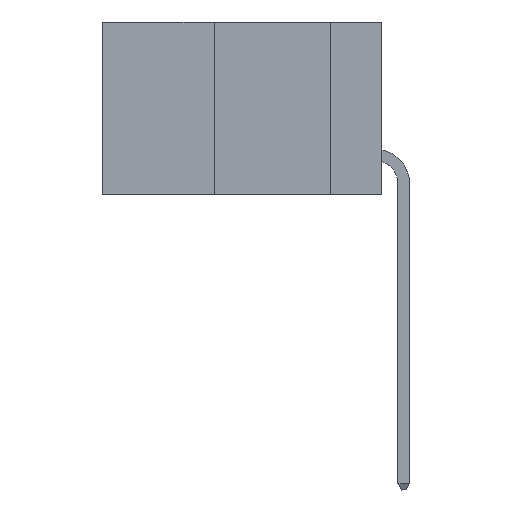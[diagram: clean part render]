
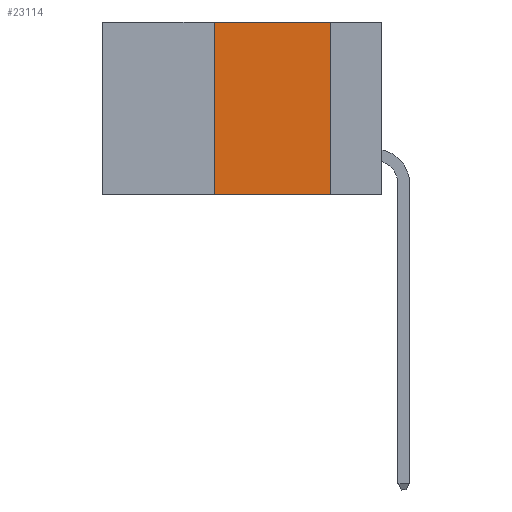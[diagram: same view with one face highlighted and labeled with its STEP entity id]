
A CAD part, left-side view. The second image highlights one B-rep face of the part: STEP entity #23114.
In plain terms, the highlighted planar face has unit normal (-1, 0, 0).
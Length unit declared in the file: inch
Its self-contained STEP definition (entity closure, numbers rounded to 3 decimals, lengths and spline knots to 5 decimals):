
#190 = DIRECTION ( 'NONE',  ( 0., -1., 0. ) ) ;
#1140 = LINE ( 'NONE', #18742, #16811 ) ;
#3027 = DIRECTION ( 'NONE',  ( 0., 0., 1. ) ) ;
#3054 = VERTEX_POINT ( 'NONE', #32082 ) ;
#3252 = AXIS2_PLACEMENT_3D ( 'NONE', #5185, #28562, #13112 ) ;
#4506 = VERTEX_POINT ( 'NONE', #28678 ) ;
#5124 = FACE_OUTER_BOUND ( 'NONE', #27759, .T. ) ;
#5164 = EDGE_CURVE ( 'NONE', #21236, #3054, #30238, .T. ) ;
#5185 = CARTESIAN_POINT ( 'NONE',  ( 0., 0.6, 0. ) ) ;
#6641 = ORIENTED_EDGE ( 'NONE', *, *, #5164, .F. ) ;
#7376 = LINE ( 'NONE', #28053, #20423 ) ;
#10482 = PLANE ( 'NONE',  #3252 ) ;
#10654 = DIRECTION ( 'NONE',  ( 0., 0., -1. ) ) ;
#11108 = ORIENTED_EDGE ( 'NONE', *, *, #32015, .F. ) ;
#13112 = DIRECTION ( 'NONE',  ( 0., 0., -1. ) ) ;
#16811 = VECTOR ( 'NONE', #3027, 39.37008 ) ;
#17406 = VECTOR ( 'NONE', #10654, 39.37008 ) ;
#17468 = EDGE_CURVE ( 'NONE', #4506, #25706, #1140, .T. ) ;
#18742 = CARTESIAN_POINT ( 'NONE',  ( 0., 0.36, 0. ) ) ;
#19627 = CARTESIAN_POINT ( 'NONE',  ( 0., 0.11, 0. ) ) ;
#19735 = LINE ( 'NONE', #31372, #33366 ) ;
#20423 = VECTOR ( 'NONE', #30622, 39.37008 ) ;
#21236 = VERTEX_POINT ( 'NONE', #19627 ) ;
#23114 = ADVANCED_FACE ( 'NONE', ( #5124 ), #10482, .F. ) ;
#24348 = EDGE_CURVE ( 'NONE', #4506, #3054, #19735, .T. ) ;
#24871 = ORIENTED_EDGE ( 'NONE', *, *, #17468, .F. ) ;
#25706 = VERTEX_POINT ( 'NONE', #33545 ) ;
#26175 = CARTESIAN_POINT ( 'NONE',  ( 0., 0.11, 0. ) ) ;
#27759 = EDGE_LOOP ( 'NONE', ( #6641, #11108, #24871, #31685 ) ) ;
#28053 = CARTESIAN_POINT ( 'NONE',  ( 0., 0.6, 0. ) ) ;
#28562 = DIRECTION ( 'NONE',  ( 1., 0., 0. ) ) ;
#28678 = CARTESIAN_POINT ( 'NONE',  ( 0., 0.36, -0.37 ) ) ;
#30238 = LINE ( 'NONE', #26175, #17406 ) ;
#30622 = DIRECTION ( 'NONE',  ( 0., -1., 0. ) ) ;
#31372 = CARTESIAN_POINT ( 'NONE',  ( 0., 0.6, -0.37 ) ) ;
#31685 = ORIENTED_EDGE ( 'NONE', *, *, #24348, .T. ) ;
#32015 = EDGE_CURVE ( 'NONE', #25706, #21236, #7376, .T. ) ;
#32082 = CARTESIAN_POINT ( 'NONE',  ( 0., 0.11, -0.37 ) ) ;
#33366 = VECTOR ( 'NONE', #190, 39.37008 ) ;
#33545 = CARTESIAN_POINT ( 'NONE',  ( 0., 0.36, 0. ) ) ;
